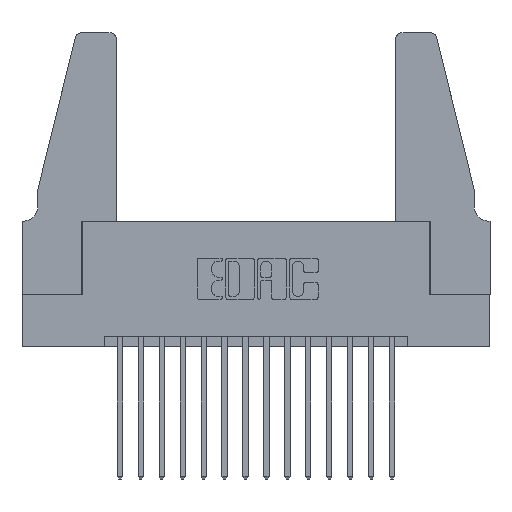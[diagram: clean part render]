
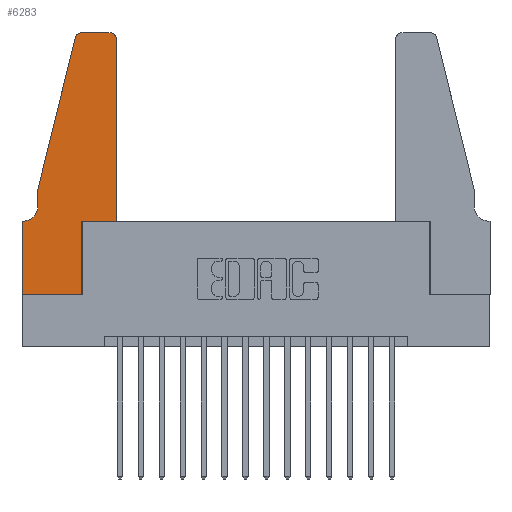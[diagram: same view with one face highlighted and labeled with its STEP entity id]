
A CAD part, top view. The second image highlights one B-rep face of the part: STEP entity #6283.
In plain terms, the highlighted planar face has unit normal (0, 0, 1).
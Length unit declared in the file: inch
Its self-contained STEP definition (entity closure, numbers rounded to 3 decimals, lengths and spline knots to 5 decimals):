
#256 = CARTESIAN_POINT ( 'NONE',  ( 0.0755, 0.5, 0.37 ) ) ;
#263 = DIRECTION ( 'NONE',  ( -0.239, -0.971, 0. ) ) ;
#489 = EDGE_CURVE ( 'NONE', #14014, #11543, #4383, .T. ) ;
#1070 = ORIENTED_EDGE ( 'NONE', *, *, #10734, .T. ) ;
#1373 = VERTEX_POINT ( 'NONE', #6149 ) ;
#1522 = DIRECTION ( 'NONE',  ( -1., 0., 0. ) ) ;
#1618 = EDGE_CURVE ( 'NONE', #1373, #14633, #10269, .T. ) ;
#1677 = CARTESIAN_POINT ( 'NONE',  ( 0.4505, 0.35, 0.37 ) ) ;
#1711 = DIRECTION ( 'NONE',  ( 0., 0., -1. ) ) ;
#1836 = DIRECTION ( 'NONE',  ( 0., -1., 0. ) ) ;
#1971 = ORIENTED_EDGE ( 'NONE', *, *, #3347, .T. ) ;
#2646 = ORIENTED_EDGE ( 'NONE', *, *, #14963, .T. ) ;
#2672 = AXIS2_PLACEMENT_3D ( 'NONE', #5375, #7899, #5433 ) ;
#2946 = CARTESIAN_POINT ( 'NONE',  ( 0.2605, 1.25, 0.37 ) ) ;
#3001 = DIRECTION ( 'NONE',  ( -1., 0., 0. ) ) ;
#3117 = CARTESIAN_POINT ( 'NONE',  ( 0., 0., 0.37 ) ) ;
#3202 = LINE ( 'NONE', #4051, #15476 ) ;
#3339 = LINE ( 'NONE', #6466, #3975 ) ;
#3347 = EDGE_CURVE ( 'NONE', #15149, #4759, #6988, .T. ) ;
#3368 = CIRCLE ( 'NONE', #5527, 0.07 ) ;
#3511 = CARTESIAN_POINT ( 'NONE',  ( 0.0755, 0.42, 0.37 ) ) ;
#3546 = VECTOR ( 'NONE', #1522, 39.37008 ) ;
#3598 = EDGE_CURVE ( 'NONE', #5552, #13567, #3368, .T. ) ;
#3875 = VECTOR ( 'NONE', #14262, 39.37008 ) ;
#3940 = ORIENTED_EDGE ( 'NONE', *, *, #3598, .T. ) ;
#3975 = VECTOR ( 'NONE', #11858, 39.37008 ) ;
#4051 = CARTESIAN_POINT ( 'NONE',  ( 0.0755, 0.35, 0.37 ) ) ;
#4146 = EDGE_CURVE ( 'NONE', #11543, #13474, #7047, .T. ) ;
#4163 = ORIENTED_EDGE ( 'NONE', *, *, #1618, .T. ) ;
#4383 = CIRCLE ( 'NONE', #2672, 0.03 ) ;
#4416 = CARTESIAN_POINT ( 'NONE',  ( 0.2865, 0.35, 0.37 ) ) ;
#4428 = CARTESIAN_POINT ( 'NONE',  ( 0.4505, 0.35, 0.37 ) ) ;
#4733 = VECTOR ( 'NONE', #263, 39.37008 ) ;
#4759 = VERTEX_POINT ( 'NONE', #256 ) ;
#4857 = VERTEX_POINT ( 'NONE', #4428 ) ;
#4930 = VECTOR ( 'NONE', #8054, 39.37008 ) ;
#4967 = LINE ( 'NONE', #9655, #14994 ) ;
#5200 = CARTESIAN_POINT ( 'NONE',  ( 0.2865, 0.35, 0.37 ) ) ;
#5375 = CARTESIAN_POINT ( 'NONE',  ( 0.4205, 1.22, 0.37 ) ) ;
#5433 = DIRECTION ( 'NONE',  ( 1., 0., 0. ) ) ;
#5440 = ORIENTED_EDGE ( 'NONE', *, *, #10326, .T. ) ;
#5506 = ORIENTED_EDGE ( 'NONE', *, *, #489, .T. ) ;
#5527 = AXIS2_PLACEMENT_3D ( 'NONE', #6900, #1711, #3001 ) ;
#5552 = VERTEX_POINT ( 'NONE', #3511 ) ;
#5890 = EDGE_CURVE ( 'NONE', #4857, #14014, #9225, .T. ) ;
#6149 = CARTESIAN_POINT ( 'NONE',  ( 0.2865, 0., 0.37 ) ) ;
#6231 = PLANE ( 'NONE',  #7273 ) ;
#6283 = ADVANCED_FACE ( 'NONE', ( #12883 ), #6231, .T. ) ;
#6287 = DIRECTION ( 'NONE',  ( 0., 0., 1. ) ) ;
#6333 = LINE ( 'NONE', #15211, #3875 ) ;
#6466 = CARTESIAN_POINT ( 'NONE',  ( 0., 0., 0.37 ) ) ;
#6632 = CARTESIAN_POINT ( 'NONE',  ( 0.0755, 0.5, 0.37 ) ) ;
#6649 = VERTEX_POINT ( 'NONE', #3117 ) ;
#6695 = CIRCLE ( 'NONE', #13233, 0.03 ) ;
#6900 = CARTESIAN_POINT ( 'NONE',  ( 0.0055, 0.42, 0.37 ) ) ;
#6988 = LINE ( 'NONE', #11898, #4733 ) ;
#7047 = LINE ( 'NONE', #2946, #3546 ) ;
#7159 = CARTESIAN_POINT ( 'NONE',  ( 0.284, 1.22, 0.37 ) ) ;
#7273 = AXIS2_PLACEMENT_3D ( 'NONE', #15488, #6287, #12906 ) ;
#7363 = CARTESIAN_POINT ( 'NONE',  ( 0.4205, 1.25, 0.37 ) ) ;
#7899 = DIRECTION ( 'NONE',  ( 0., 0., 1. ) ) ;
#8054 = DIRECTION ( 'NONE',  ( 0., 1., 0. ) ) ;
#8356 = DIRECTION ( 'NONE',  ( 0., 0., 1. ) ) ;
#8630 = EDGE_CURVE ( 'NONE', #4759, #5552, #9928, .T. ) ;
#8897 = ORIENTED_EDGE ( 'NONE', *, *, #5890, .T. ) ;
#9225 = LINE ( 'NONE', #1677, #4930 ) ;
#9655 = CARTESIAN_POINT ( 'NONE',  ( 0., 0., 0.37 ) ) ;
#9852 = ORIENTED_EDGE ( 'NONE', *, *, #13276, .T. ) ;
#9928 = LINE ( 'NONE', #6632, #16296 ) ;
#9976 = CARTESIAN_POINT ( 'NONE',  ( 0.0055, 0.35, 0.37 ) ) ;
#10269 = LINE ( 'NONE', #5200, #16036 ) ;
#10326 = EDGE_CURVE ( 'NONE', #13474, #15149, #6695, .T. ) ;
#10390 = DIRECTION ( 'NONE',  ( 0., 1., 0. ) ) ;
#10734 = EDGE_CURVE ( 'NONE', #13567, #11038, #3202, .T. ) ;
#10927 = EDGE_LOOP ( 'NONE', ( #15410, #5440, #1971, #11984, #3940, #1070, #9852, #14180, #4163, #2646, #8897, #5506 ) ) ;
#11038 = VERTEX_POINT ( 'NONE', #14144 ) ;
#11543 = VERTEX_POINT ( 'NONE', #7363 ) ;
#11858 = DIRECTION ( 'NONE',  ( 1., 0., 0. ) ) ;
#11898 = CARTESIAN_POINT ( 'NONE',  ( 0.0755, 0.5, 0.37 ) ) ;
#11984 = ORIENTED_EDGE ( 'NONE', *, *, #8630, .T. ) ;
#12082 = CARTESIAN_POINT ( 'NONE',  ( 0.25487, 1.22718, 0.37 ) ) ;
#12157 = EDGE_CURVE ( 'NONE', #6649, #1373, #3339, .T. ) ;
#12883 = FACE_OUTER_BOUND ( 'NONE', #10927, .T. ) ;
#12906 = DIRECTION ( 'NONE',  ( 1., 0., 0. ) ) ;
#13197 = DIRECTION ( 'NONE',  ( -1., 0., 0. ) ) ;
#13233 = AXIS2_PLACEMENT_3D ( 'NONE', #7159, #8356, #16336 ) ;
#13276 = EDGE_CURVE ( 'NONE', #11038, #6649, #4967, .T. ) ;
#13474 = VERTEX_POINT ( 'NONE', #14066 ) ;
#13567 = VERTEX_POINT ( 'NONE', #9976 ) ;
#14014 = VERTEX_POINT ( 'NONE', #16337 ) ;
#14066 = CARTESIAN_POINT ( 'NONE',  ( 0.284, 1.25, 0.37 ) ) ;
#14144 = CARTESIAN_POINT ( 'NONE',  ( 0., 0.35, 0.37 ) ) ;
#14180 = ORIENTED_EDGE ( 'NONE', *, *, #12157, .T. ) ;
#14262 = DIRECTION ( 'NONE',  ( 1., 0., 0. ) ) ;
#14512 = DIRECTION ( 'NONE',  ( 0., -1., 0. ) ) ;
#14633 = VERTEX_POINT ( 'NONE', #4416 ) ;
#14963 = EDGE_CURVE ( 'NONE', #14633, #4857, #6333, .T. ) ;
#14994 = VECTOR ( 'NONE', #1836, 39.37008 ) ;
#15149 = VERTEX_POINT ( 'NONE', #12082 ) ;
#15211 = CARTESIAN_POINT ( 'NONE',  ( 0.4505, 0.35, 0.37 ) ) ;
#15410 = ORIENTED_EDGE ( 'NONE', *, *, #4146, .T. ) ;
#15476 = VECTOR ( 'NONE', #13197, 39.37008 ) ;
#15488 = CARTESIAN_POINT ( 'NONE',  ( 0., 0.35, 0.37 ) ) ;
#16036 = VECTOR ( 'NONE', #10390, 39.37008 ) ;
#16296 = VECTOR ( 'NONE', #14512, 39.37008 ) ;
#16336 = DIRECTION ( 'NONE',  ( 1., 0., 0. ) ) ;
#16337 = CARTESIAN_POINT ( 'NONE',  ( 0.4505, 1.22, 0.37 ) ) ;
